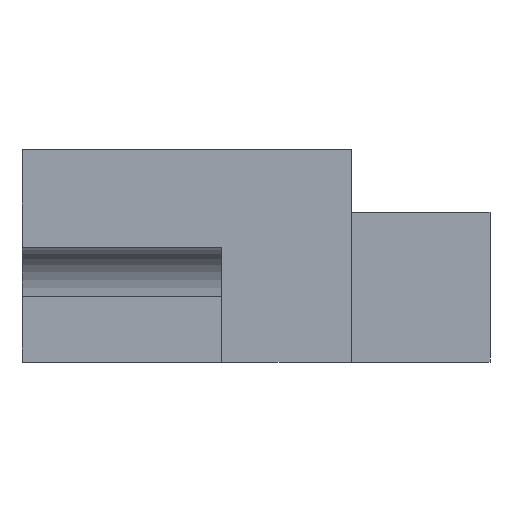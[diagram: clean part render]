
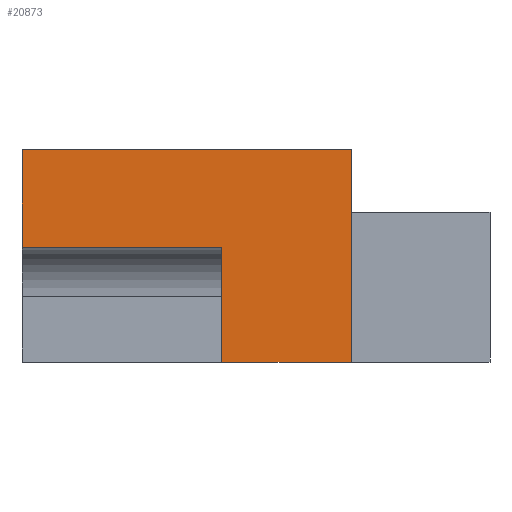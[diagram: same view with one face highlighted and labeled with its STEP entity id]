
A CAD part, left-side view. The second image highlights one B-rep face of the part: STEP entity #20873.
In plain terms, the highlighted planar face has unit normal (-1, 0, 0).
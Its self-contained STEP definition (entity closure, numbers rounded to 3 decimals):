
#418 = VERTEX_POINT ( 'NONE', #844 ) ;
#450 = EDGE_CURVE ( 'NONE', #16181, #3088, #3631, .T. ) ;
#844 = CARTESIAN_POINT ( 'NONE',  ( 0., 8.255, -13.487 ) ) ;
#922 = CARTESIAN_POINT ( 'NONE',  ( 0., 20.955, 0. ) ) ;
#1155 = DIRECTION ( 'NONE',  ( 0., 0., -1. ) ) ;
#1257 = CARTESIAN_POINT ( 'NONE',  ( 0., 0., 0. ) ) ;
#1352 = ORIENTED_EDGE ( 'NONE', *, *, #4509, .F. ) ;
#1949 = EDGE_CURVE ( 'NONE', #3088, #14003, #19540, .T. ) ;
#2374 = CARTESIAN_POINT ( 'NONE',  ( 0., 20.955, -6.172 ) ) ;
#2781 = CARTESIAN_POINT ( 'NONE',  ( 0., 0., -13.487 ) ) ;
#3088 = VERTEX_POINT ( 'NONE', #922 ) ;
#3190 = ORIENTED_EDGE ( 'NONE', *, *, #7818, .F. ) ;
#3282 = EDGE_CURVE ( 'NONE', #6425, #16181, #7987, .T. ) ;
#3631 = LINE ( 'NONE', #7208, #15907 ) ;
#4007 = CARTESIAN_POINT ( 'NONE',  ( 0., 8.255, -6.172 ) ) ;
#4309 = DIRECTION ( 'NONE',  ( 0., -1., 0. ) ) ;
#4463 = LINE ( 'NONE', #12865, #19318 ) ;
#4509 = EDGE_CURVE ( 'NONE', #12931, #418, #11275, .T. ) ;
#6063 = CARTESIAN_POINT ( 'NONE',  ( 0., 8.255, -6.172 ) ) ;
#6425 = VERTEX_POINT ( 'NONE', #6063 ) ;
#7208 = CARTESIAN_POINT ( 'NONE',  ( 0., 20.955, -13.487 ) ) ;
#7668 = AXIS2_PLACEMENT_3D ( 'NONE', #1257, #14429, #16045 ) ;
#7685 = CARTESIAN_POINT ( 'NONE',  ( 0., 11.506, 0. ) ) ;
#7818 = EDGE_CURVE ( 'NONE', #418, #6425, #4463, .T. ) ;
#7987 = LINE ( 'NONE', #4007, #10037 ) ;
#9003 = DIRECTION ( 'NONE',  ( 0., 0., 1. ) ) ;
#10037 = VECTOR ( 'NONE', #12028, 1000. ) ;
#11275 = LINE ( 'NONE', #17726, #12281 ) ;
#11429 = ORIENTED_EDGE ( 'NONE', *, *, #14362, .F. ) ;
#12028 = DIRECTION ( 'NONE',  ( 0., 1., 0. ) ) ;
#12281 = VECTOR ( 'NONE', #14575, 1000. ) ;
#12865 = CARTESIAN_POINT ( 'NONE',  ( 0., 8.255, -13.487 ) ) ;
#12931 = VERTEX_POINT ( 'NONE', #2781 ) ;
#13649 = VECTOR ( 'NONE', #4309, 1000. ) ;
#14003 = VERTEX_POINT ( 'NONE', #14548 ) ;
#14362 = EDGE_CURVE ( 'NONE', #14003, #12931, #19697, .T. ) ;
#14429 = DIRECTION ( 'NONE',  ( 1., 0., 0. ) ) ;
#14527 = ORIENTED_EDGE ( 'NONE', *, *, #1949, .F. ) ;
#14548 = CARTESIAN_POINT ( 'NONE',  ( 0., 0., 0. ) ) ;
#14575 = DIRECTION ( 'NONE',  ( 0., 1., 0. ) ) ;
#15442 = PLANE ( 'NONE',  #7668 ) ;
#15907 = VECTOR ( 'NONE', #9003, 1000. ) ;
#16045 = DIRECTION ( 'NONE',  ( 0., 0., -1. ) ) ;
#16181 = VERTEX_POINT ( 'NONE', #2374 ) ;
#16277 = DIRECTION ( 'NONE',  ( 0., 0., 1. ) ) ;
#16617 = FACE_OUTER_BOUND ( 'NONE', #17497, .T. ) ;
#16941 = CARTESIAN_POINT ( 'NONE',  ( 0., 0., 0. ) ) ;
#17497 = EDGE_LOOP ( 'NONE', ( #1352, #11429, #14527, #20152, #21014, #3190 ) ) ;
#17726 = CARTESIAN_POINT ( 'NONE',  ( 0., -8.814, -13.487 ) ) ;
#19318 = VECTOR ( 'NONE', #16277, 1000. ) ;
#19540 = LINE ( 'NONE', #7685, #13649 ) ;
#19697 = LINE ( 'NONE', #16941, #21216 ) ;
#20152 = ORIENTED_EDGE ( 'NONE', *, *, #450, .F. ) ;
#20873 = ADVANCED_FACE ( 'NONE', ( #16617 ), #15442, .F. ) ;
#21014 = ORIENTED_EDGE ( 'NONE', *, *, #3282, .F. ) ;
#21216 = VECTOR ( 'NONE', #1155, 1000. ) ;
